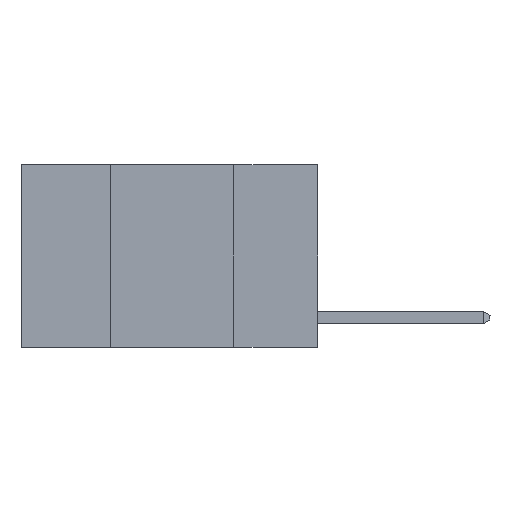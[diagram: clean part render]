
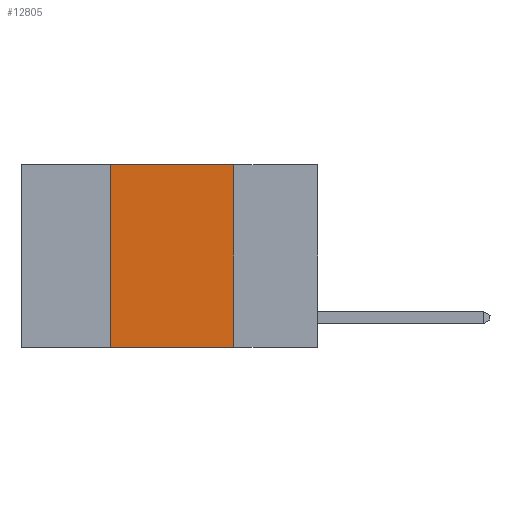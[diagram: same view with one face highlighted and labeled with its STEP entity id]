
A CAD part, left-side view. The second image highlights one B-rep face of the part: STEP entity #12805.
In plain terms, the highlighted planar face has unit normal (-1, 0, 0).
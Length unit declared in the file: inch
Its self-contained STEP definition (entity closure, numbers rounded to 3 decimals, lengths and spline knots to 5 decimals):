
#141 = DIRECTION ( 'NONE',  ( 0., 0., 1. ) ) ;
#579 = ORIENTED_EDGE ( 'NONE', *, *, #6327, .F. ) ;
#739 = CARTESIAN_POINT ( 'NONE',  ( 0., 0.17, 0. ) ) ;
#969 = DIRECTION ( 'NONE',  ( 0., 0., -1. ) ) ;
#2078 = CARTESIAN_POINT ( 'NONE',  ( 0., 0.17, 0. ) ) ;
#3669 = CARTESIAN_POINT ( 'NONE',  ( 0., 0.42, -0.37 ) ) ;
#3781 = EDGE_CURVE ( 'NONE', #15197, #4434, #5989, .T. ) ;
#4137 = EDGE_CURVE ( 'NONE', #14339, #4434, #13559, .T. ) ;
#4155 = VERTEX_POINT ( 'NONE', #27140 ) ;
#4434 = VERTEX_POINT ( 'NONE', #7044 ) ;
#4667 = ORIENTED_EDGE ( 'NONE', *, *, #19603, .F. ) ;
#5352 = VECTOR ( 'NONE', #25876, 39.37008 ) ;
#5989 = LINE ( 'NONE', #739, #5352 ) ;
#6174 = ORIENTED_EDGE ( 'NONE', *, *, #4137, .T. ) ;
#6327 = EDGE_CURVE ( 'NONE', #14339, #4155, #22803, .T. ) ;
#7044 = CARTESIAN_POINT ( 'NONE',  ( 0., 0.17, -0.37 ) ) ;
#8269 = DIRECTION ( 'NONE',  ( 0., -1., 0. ) ) ;
#9655 = LINE ( 'NONE', #25060, #20194 ) ;
#10240 = ORIENTED_EDGE ( 'NONE', *, *, #3781, .F. ) ;
#10287 = CARTESIAN_POINT ( 'NONE',  ( 0., 0.6, -0.37 ) ) ;
#11468 = PLANE ( 'NONE',  #19424 ) ;
#12805 = ADVANCED_FACE ( 'NONE', ( #23548 ), #11468, .F. ) ;
#12887 = VECTOR ( 'NONE', #26959, 39.37008 ) ;
#13559 = LINE ( 'NONE', #10287, #12887 ) ;
#13594 = DIRECTION ( 'NONE',  ( 1., 0., 0. ) ) ;
#14339 = VERTEX_POINT ( 'NONE', #3669 ) ;
#15197 = VERTEX_POINT ( 'NONE', #2078 ) ;
#16551 = VECTOR ( 'NONE', #141, 39.37008 ) ;
#17410 = EDGE_LOOP ( 'NONE', ( #10240, #4667, #579, #6174 ) ) ;
#18917 = CARTESIAN_POINT ( 'NONE',  ( 0., 0.42, 0. ) ) ;
#19424 = AXIS2_PLACEMENT_3D ( 'NONE', #23943, #13594, #969 ) ;
#19603 = EDGE_CURVE ( 'NONE', #4155, #15197, #9655, .T. ) ;
#20194 = VECTOR ( 'NONE', #8269, 39.37008 ) ;
#22803 = LINE ( 'NONE', #18917, #16551 ) ;
#23548 = FACE_OUTER_BOUND ( 'NONE', #17410, .T. ) ;
#23943 = CARTESIAN_POINT ( 'NONE',  ( 0., 0.6, 0. ) ) ;
#25060 = CARTESIAN_POINT ( 'NONE',  ( 0., 0.6, 0. ) ) ;
#25876 = DIRECTION ( 'NONE',  ( 0., 0., -1. ) ) ;
#26959 = DIRECTION ( 'NONE',  ( 0., -1., 0. ) ) ;
#27140 = CARTESIAN_POINT ( 'NONE',  ( 0., 0.42, 0. ) ) ;
